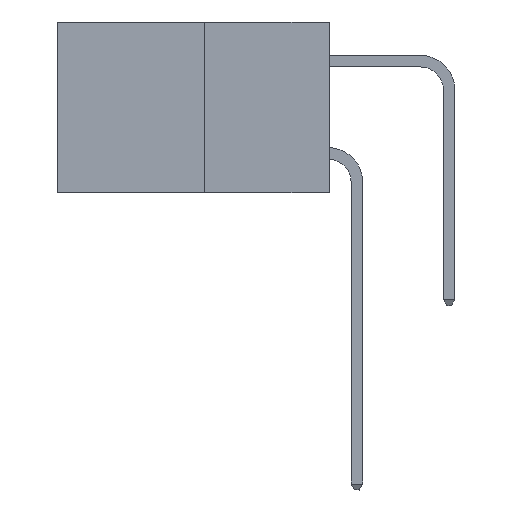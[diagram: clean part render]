
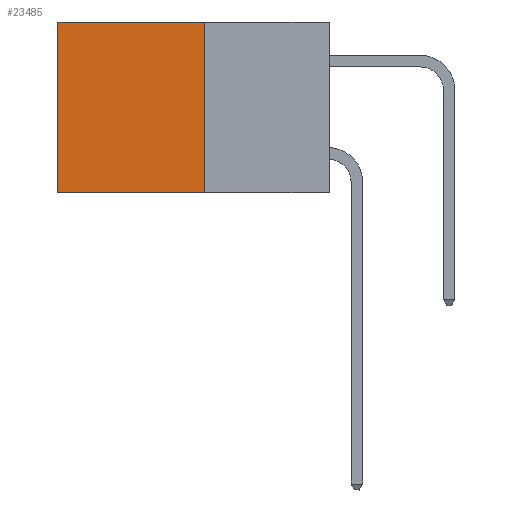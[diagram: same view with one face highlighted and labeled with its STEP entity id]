
A CAD part, left-side view. The second image highlights one B-rep face of the part: STEP entity #23485.
In plain terms, the highlighted planar face has unit normal (-1, 0, 0).
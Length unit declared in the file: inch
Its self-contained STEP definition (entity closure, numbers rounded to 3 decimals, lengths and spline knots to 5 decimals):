
#21 = VERTEX_POINT ( 'NONE', #9180 ) ;
#95 = CARTESIAN_POINT ( 'NONE',  ( 0.277, 0.59, -0.37 ) ) ;
#184 = DIRECTION ( 'NONE',  ( 0., 0., -1. ) ) ;
#408 = EDGE_CURVE ( 'NONE', #17097, #28744, #7307, .T. ) ;
#2374 = ORIENTED_EDGE ( 'NONE', *, *, #14370, .F. ) ;
#4704 = DIRECTION ( 'NONE',  ( 1., 0., 0. ) ) ;
#4939 = CARTESIAN_POINT ( 'NONE',  ( 0.277, 0.27, 0. ) ) ;
#7307 = LINE ( 'NONE', #4939, #19206 ) ;
#7698 = CARTESIAN_POINT ( 'NONE',  ( 0.277, 0.27, 0. ) ) ;
#9180 = CARTESIAN_POINT ( 'NONE',  ( 0.277, 0.27, -0.37 ) ) ;
#10155 = EDGE_CURVE ( 'NONE', #28744, #12590, #19097, .T. ) ;
#10243 = EDGE_CURVE ( 'NONE', #17097, #21, #30176, .T. ) ;
#11746 = PLANE ( 'NONE',  #30656 ) ;
#12590 = VERTEX_POINT ( 'NONE', #18397 ) ;
#12776 = VECTOR ( 'NONE', #184, 39.37008 ) ;
#13172 = ORIENTED_EDGE ( 'NONE', *, *, #408, .T. ) ;
#13354 = ORIENTED_EDGE ( 'NONE', *, *, #10243, .F. ) ;
#14370 = EDGE_CURVE ( 'NONE', #21, #12590, #23022, .T. ) ;
#15509 = DIRECTION ( 'NONE',  ( 0., 1., 0. ) ) ;
#17097 = VERTEX_POINT ( 'NONE', #7698 ) ;
#17644 = VECTOR ( 'NONE', #21733, 39.37008 ) ;
#18397 = CARTESIAN_POINT ( 'NONE',  ( 0.277, 0.59, -0.37 ) ) ;
#18953 = CARTESIAN_POINT ( 'NONE',  ( 0.277, 0.27, -0.37 ) ) ;
#19097 = LINE ( 'NONE', #95, #12776 ) ;
#19206 = VECTOR ( 'NONE', #28227, 39.37008 ) ;
#21304 = DIRECTION ( 'NONE',  ( 0., 0., -1. ) ) ;
#21733 = DIRECTION ( 'NONE',  ( 0., 0., -1. ) ) ;
#22422 = ORIENTED_EDGE ( 'NONE', *, *, #10155, .T. ) ;
#23022 = LINE ( 'NONE', #29662, #30057 ) ;
#23200 = FACE_OUTER_BOUND ( 'NONE', #30246, .T. ) ;
#23485 = ADVANCED_FACE ( 'NONE', ( #23200 ), #11746, .F. ) ;
#26134 = CARTESIAN_POINT ( 'NONE',  ( 0.277, 0.59, 0. ) ) ;
#28227 = DIRECTION ( 'NONE',  ( 0., 1., 0. ) ) ;
#28744 = VERTEX_POINT ( 'NONE', #26134 ) ;
#28873 = CARTESIAN_POINT ( 'NONE',  ( 0.277, 0.27, -0.37 ) ) ;
#29662 = CARTESIAN_POINT ( 'NONE',  ( 0.277, 0.27, -0.37 ) ) ;
#30057 = VECTOR ( 'NONE', #15509, 39.37008 ) ;
#30176 = LINE ( 'NONE', #28873, #17644 ) ;
#30246 = EDGE_LOOP ( 'NONE', ( #22422, #2374, #13354, #13172 ) ) ;
#30656 = AXIS2_PLACEMENT_3D ( 'NONE', #18953, #4704, #21304 ) ;
